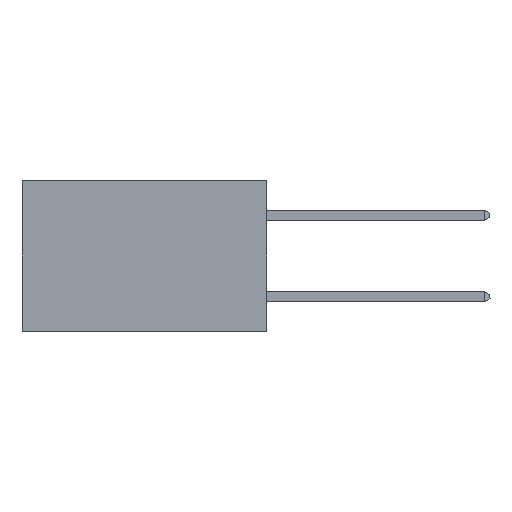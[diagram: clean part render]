
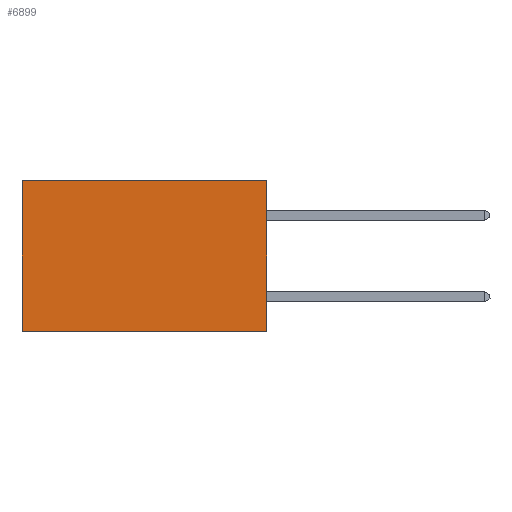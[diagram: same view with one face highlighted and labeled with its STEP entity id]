
A CAD part, left-side view. The second image highlights one B-rep face of the part: STEP entity #6899.
In plain terms, the highlighted planar face has unit normal (-1, 0, 0).
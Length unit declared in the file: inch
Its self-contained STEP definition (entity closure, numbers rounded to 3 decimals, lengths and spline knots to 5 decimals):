
#88 = LINE ( 'NONE', #12002, #12033 ) ;
#194 = ORIENTED_EDGE ( 'NONE', *, *, #11002, .T. ) ;
#634 = ORIENTED_EDGE ( 'NONE', *, *, #1597, .T. ) ;
#919 = DIRECTION ( 'NONE',  ( 0., 0., -1. ) ) ;
#1289 = CARTESIAN_POINT ( 'NONE',  ( 0.2875, 0., 0. ) ) ;
#1597 = EDGE_CURVE ( 'NONE', #15069, #13422, #13839, .T. ) ;
#1749 = FACE_OUTER_BOUND ( 'NONE', #6711, .T. ) ;
#1851 = VECTOR ( 'NONE', #5631, 39.37008 ) ;
#1908 = EDGE_CURVE ( 'NONE', #15069, #6064, #7295, .T. ) ;
#3821 = CARTESIAN_POINT ( 'NONE',  ( 0.2875, 0.6, 0. ) ) ;
#4598 = PLANE ( 'NONE',  #10335 ) ;
#5519 = CARTESIAN_POINT ( 'NONE',  ( 0.2875, 0., 0. ) ) ;
#5631 = DIRECTION ( 'NONE',  ( 0., 1., 0. ) ) ;
#6064 = VERTEX_POINT ( 'NONE', #7898 ) ;
#6711 = EDGE_LOOP ( 'NONE', ( #194, #16266, #16235, #634 ) ) ;
#6812 = VERTEX_POINT ( 'NONE', #12164 ) ;
#6858 = CARTESIAN_POINT ( 'NONE',  ( 0.2875, 0., -0.37 ) ) ;
#6899 = ADVANCED_FACE ( 'NONE', ( #1749 ), #4598, .F. ) ;
#7295 = LINE ( 'NONE', #1289, #11667 ) ;
#7579 = DIRECTION ( 'NONE',  ( 0., 0., -1. ) ) ;
#7898 = CARTESIAN_POINT ( 'NONE',  ( 0.2875, 0., -0.37 ) ) ;
#10335 = AXIS2_PLACEMENT_3D ( 'NONE', #12326, #13469, #919 ) ;
#10652 = DIRECTION ( 'NONE',  ( 0., 1., 0. ) ) ;
#11002 = EDGE_CURVE ( 'NONE', #13422, #6812, #88, .T. ) ;
#11667 = VECTOR ( 'NONE', #7579, 39.37008 ) ;
#11720 = EDGE_CURVE ( 'NONE', #6064, #6812, #12189, .T. ) ;
#11940 = DIRECTION ( 'NONE',  ( 0., 0., -1. ) ) ;
#12002 = CARTESIAN_POINT ( 'NONE',  ( 0.2875, 0.6, 0. ) ) ;
#12033 = VECTOR ( 'NONE', #11940, 39.37008 ) ;
#12164 = CARTESIAN_POINT ( 'NONE',  ( 0.2875, 0.6, -0.37 ) ) ;
#12189 = LINE ( 'NONE', #6858, #1851 ) ;
#12326 = CARTESIAN_POINT ( 'NONE',  ( 0.2875, 0., 0. ) ) ;
#13422 = VERTEX_POINT ( 'NONE', #3821 ) ;
#13448 = VECTOR ( 'NONE', #10652, 39.37008 ) ;
#13469 = DIRECTION ( 'NONE',  ( 1., 0., 0. ) ) ;
#13839 = LINE ( 'NONE', #5519, #13448 ) ;
#13881 = CARTESIAN_POINT ( 'NONE',  ( 0.2875, 0., 0. ) ) ;
#15069 = VERTEX_POINT ( 'NONE', #13881 ) ;
#16235 = ORIENTED_EDGE ( 'NONE', *, *, #1908, .F. ) ;
#16266 = ORIENTED_EDGE ( 'NONE', *, *, #11720, .F. ) ;
